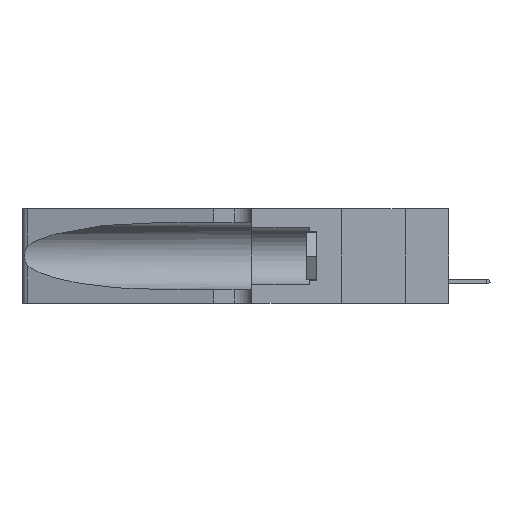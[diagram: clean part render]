
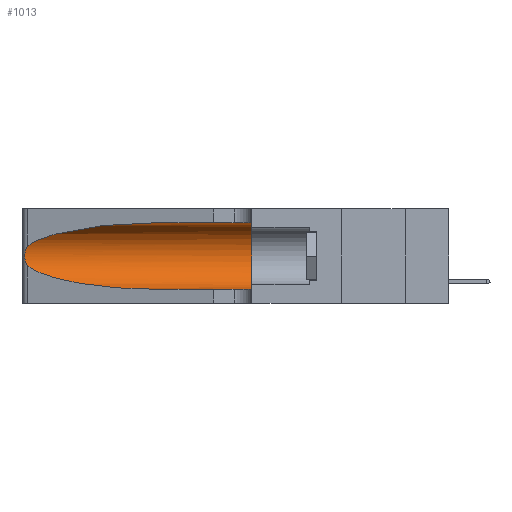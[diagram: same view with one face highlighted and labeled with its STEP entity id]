
A CAD part, left-side view. The second image highlights one B-rep face of the part: STEP entity #1013.
In plain terms, the highlighted cylindrical face has radius 3.308 mm (diameter 6.617 mm), a partial arc.
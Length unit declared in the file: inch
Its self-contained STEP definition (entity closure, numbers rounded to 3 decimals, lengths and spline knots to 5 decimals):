
#264 = CARTESIAN_POINT ( 'NONE',  ( 0.1305, 1.61858, 0.05475 ) ) ;
#951 = ORIENTED_EDGE ( 'NONE', *, *, #20871, .F. ) ;
#1013 = ADVANCED_FACE ( 'NONE', ( #8592 ), #15490, .F. ) ;
#1397 = CARTESIAN_POINT ( 'NONE',  ( 0.25555, 1.22994, 0.2215 ) ) ;
#1660 = CARTESIAN_POINT ( 'NONE',  ( 0.26017, 1.23833, 0.17102 ) ) ;
#2238 = VERTEX_POINT ( 'NONE', #7717 ) ;
#3582 = CARTESIAN_POINT ( 'NONE',  ( 0.18966, 0.96281, 0.31525 ) ) ;
#3614 = EDGE_CURVE ( 'NONE', #6777, #20175, #4358, .T. ) ;
#3752 = CARTESIAN_POINT ( 'NONE',  ( 0.26075, 1.23896, 0.19203 ) ) ;
#3881 = ORIENTED_EDGE ( 'NONE', *, *, #24644, .T. ) ;
#4358 =( BOUNDED_CURVE ( )  B_SPLINE_CURVE ( 3, ( #10334, #21967, #10157, #8112 ),
 .UNSPECIFIED., .F., .F. ) 
 B_SPLINE_CURVE_WITH_KNOTS ( ( 4, 4 ),
 ( 3.44316, 4.71239 ),
 .UNSPECIFIED. ) 
 CURVE ( )  GEOMETRIC_REPRESENTATION_ITEM ( )  RATIONAL_B_SPLINE_CURVE ( ( 1., 0.87, 0.87, 1. ) ) 
 REPRESENTATION_ITEM ( '' )  );
#5414 = CARTESIAN_POINT ( 'NONE',  ( 0.25787, 1.23484, 0.2124 ) ) ;
#6145 = DIRECTION ( 'NONE',  ( 0., -1., 0. ) ) ;
#6446 = LINE ( 'NONE', #23568, #25877 ) ;
#6489 = ORIENTED_EDGE ( 'NONE', *, *, #7721, .T. ) ;
#6777 = VERTEX_POINT ( 'NONE', #16689 ) ;
#7579 = VERTEX_POINT ( 'NONE', #17074 ) ;
#7690 = CARTESIAN_POINT ( 'NONE',  ( 0.25639, 1.23186, 0.15144 ) ) ;
#7717 = CARTESIAN_POINT ( 'NONE',  ( 0.25487, 1.22718, 0.22369 ) ) ;
#7721 = EDGE_CURVE ( 'NONE', #20175, #13991, #20872, .T. ) ;
#7774 = CARTESIAN_POINT ( 'NONE',  ( 0.25639, 1.23184, 0.21858 ) ) ;
#8112 = CARTESIAN_POINT ( 'NONE',  ( 0.1305, 0.72297, 0.05475 ) ) ;
#8579 = DIRECTION ( 'NONE',  ( 0., 1., 0. ) ) ;
#8592 = FACE_OUTER_BOUND ( 'NONE', #9570, .T. ) ;
#9086 = EDGE_CURVE ( 'NONE', #12514, #2238, #19620, .T. ) ;
#9453 = DIRECTION ( 'NONE',  ( 0., -1., 0. ) ) ;
#9479 = EDGE_CURVE ( 'NONE', #12514, #7579, #6446, .T. ) ;
#9570 = EDGE_LOOP ( 'NONE', ( #11080, #3881, #19552, #6489, #951, #12754 ) ) ;
#9644 = CARTESIAN_POINT ( 'NONE',  ( 0.25555, 1.22993, 0.14849 ) ) ;
#10157 = CARTESIAN_POINT ( 'NONE',  ( 0.18966, 0.96281, 0.05475 ) ) ;
#10334 = CARTESIAN_POINT ( 'NONE',  ( 0.25487, 1.22718, 0.14631 ) ) ;
#11080 = ORIENTED_EDGE ( 'NONE', *, *, #9086, .T. ) ;
#11669 = CARTESIAN_POINT ( 'NONE',  ( 0.25487, 1.22718, 0.14631 ) ) ;
#12166 = CARTESIAN_POINT ( 'NONE',  ( 0.1305, 0.72297, 0.05475 ) ) ;
#12514 = VERTEX_POINT ( 'NONE', #20572 ) ;
#12754 = ORIENTED_EDGE ( 'NONE', *, *, #9479, .F. ) ;
#13440 = CARTESIAN_POINT ( 'NONE',  ( 0.2373, 1.15595, 0.28018 ) ) ;
#13597 = DIRECTION ( 'NONE',  ( 0., -1., 0. ) ) ;
#13687 = B_SPLINE_CURVE_WITH_KNOTS ( 'NONE', 3,
 ( #19109, #1397, #7774, #5414, #15411, #21647, #3752, #13759, #1660, #19715, #23582, #7690, #9644, #11669 ),
 .UNSPECIFIED., .F., .F.,
 ( 4, 2, 2, 2, 2, 2, 4 ),
 ( 0., 0.00027, 0.00053, 0.00107, 0.0016, 0.00187, 0.00214 ),
 .UNSPECIFIED. ) ;
#13759 = CARTESIAN_POINT ( 'NONE',  ( 0.26075, 1.23896, 0.178 ) ) ;
#13991 = VERTEX_POINT ( 'NONE', #17560 ) ;
#14746 = CARTESIAN_POINT ( 'NONE',  ( 0.1305, 0.35, 0.185 ) ) ;
#14984 = AXIS2_PLACEMENT_3D ( 'NONE', #17540, #13597, #23837 ) ;
#15411 = CARTESIAN_POINT ( 'NONE',  ( 0.25854, 1.2359, 0.20912 ) ) ;
#15490 = CYLINDRICAL_SURFACE ( 'NONE', #14984, 0.13025 ) ;
#15528 = VECTOR ( 'NONE', #6145, 39.37008 ) ;
#16689 = CARTESIAN_POINT ( 'NONE',  ( 0.25487, 1.22718, 0.14631 ) ) ;
#17074 = CARTESIAN_POINT ( 'NONE',  ( 0.1305, 0.35, 0.31525 ) ) ;
#17540 = CARTESIAN_POINT ( 'NONE',  ( 0.1305, 1.61858, 0.185 ) ) ;
#17560 = CARTESIAN_POINT ( 'NONE',  ( 0.1305, 0.35, 0.05475 ) ) ;
#17669 = AXIS2_PLACEMENT_3D ( 'NONE', #14746, #8579, #22147 ) ;
#19032 = CARTESIAN_POINT ( 'NONE',  ( 0.1305, 0.72297, 0.31525 ) ) ;
#19109 = CARTESIAN_POINT ( 'NONE',  ( 0.25487, 1.22718, 0.22369 ) ) ;
#19552 = ORIENTED_EDGE ( 'NONE', *, *, #3614, .T. ) ;
#19620 =( BOUNDED_CURVE ( )  B_SPLINE_CURVE ( 3, ( #19032, #3582, #13440, #21485 ),
 .UNSPECIFIED., .F., .F. ) 
 B_SPLINE_CURVE_WITH_KNOTS ( ( 4, 4 ),
 ( 1.5708, 2.84003 ),
 .UNSPECIFIED. ) 
 CURVE ( )  GEOMETRIC_REPRESENTATION_ITEM ( )  RATIONAL_B_SPLINE_CURVE ( ( 1., 0.87, 0.87, 1. ) ) 
 REPRESENTATION_ITEM ( '' )  );
#19715 = CARTESIAN_POINT ( 'NONE',  ( 0.25856, 1.23593, 0.16098 ) ) ;
#20175 = VERTEX_POINT ( 'NONE', #12166 ) ;
#20572 = CARTESIAN_POINT ( 'NONE',  ( 0.1305, 0.72297, 0.31525 ) ) ;
#20871 = EDGE_CURVE ( 'NONE', #7579, #13991, #21916, .T. ) ;
#20872 = LINE ( 'NONE', #264, #15528 ) ;
#21485 = CARTESIAN_POINT ( 'NONE',  ( 0.25487, 1.22718, 0.22369 ) ) ;
#21647 = CARTESIAN_POINT ( 'NONE',  ( 0.26018, 1.23835, 0.19895 ) ) ;
#21916 = CIRCLE ( 'NONE', #17669, 0.13025 ) ;
#21967 = CARTESIAN_POINT ( 'NONE',  ( 0.2373, 1.15595, 0.08982 ) ) ;
#22147 = DIRECTION ( 'NONE',  ( 0., 0., 1. ) ) ;
#23568 = CARTESIAN_POINT ( 'NONE',  ( 0.1305, 1.61858, 0.31525 ) ) ;
#23582 = CARTESIAN_POINT ( 'NONE',  ( 0.25789, 1.23486, 0.15765 ) ) ;
#23837 = DIRECTION ( 'NONE',  ( 0., 0., -1. ) ) ;
#24644 = EDGE_CURVE ( 'NONE', #2238, #6777, #13687, .T. ) ;
#25877 = VECTOR ( 'NONE', #9453, 39.37008 ) ;
